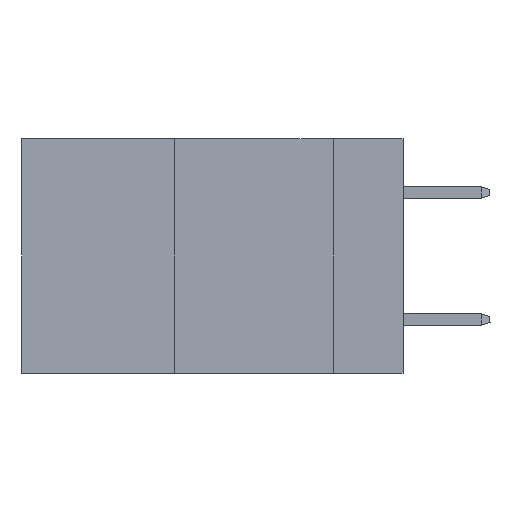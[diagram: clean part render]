
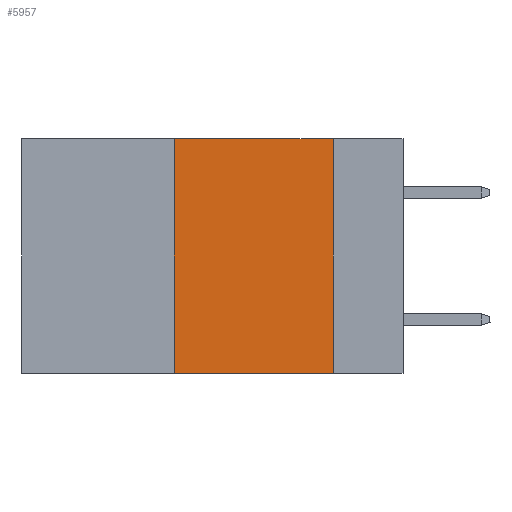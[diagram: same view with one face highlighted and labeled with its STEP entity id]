
A CAD part, left-side view. The second image highlights one B-rep face of the part: STEP entity #5957.
In plain terms, the highlighted planar face has unit normal (-1, 0, 0).
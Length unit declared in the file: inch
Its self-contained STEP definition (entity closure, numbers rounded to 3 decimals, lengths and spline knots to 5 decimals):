
#742 = CARTESIAN_POINT ( 'NONE',  ( 0., 0.6, -0.37 ) ) ;
#1434 = EDGE_CURVE ( 'NONE', #24306, #23493, #7871, .T. ) ;
#1919 = CARTESIAN_POINT ( 'NONE',  ( 0., 0.11, -0.37 ) ) ;
#2840 = DIRECTION ( 'NONE',  ( 0., -1., 0. ) ) ;
#4741 = DIRECTION ( 'NONE',  ( 1., 0., 0. ) ) ;
#4918 = CARTESIAN_POINT ( 'NONE',  ( 0., 0.11, 0. ) ) ;
#5442 = ORIENTED_EDGE ( 'NONE', *, *, #32337, .F. ) ;
#5957 = ADVANCED_FACE ( 'NONE', ( #20159 ), #32544, .F. ) ;
#7871 = LINE ( 'NONE', #13069, #31113 ) ;
#9867 = AXIS2_PLACEMENT_3D ( 'NONE', #14803, #4741, #20486 ) ;
#10451 = DIRECTION ( 'NONE',  ( 0., -1., 0. ) ) ;
#11065 = CARTESIAN_POINT ( 'NONE',  ( 0., 0.11, 0. ) ) ;
#12007 = EDGE_CURVE ( 'NONE', #17244, #28889, #23196, .T. ) ;
#13069 = CARTESIAN_POINT ( 'NONE',  ( 0., 0.6, 0. ) ) ;
#13673 = DIRECTION ( 'NONE',  ( 0., 0., 1. ) ) ;
#14803 = CARTESIAN_POINT ( 'NONE',  ( 0., 0.6, 0. ) ) ;
#17109 = ORIENTED_EDGE ( 'NONE', *, *, #17417, .F. ) ;
#17244 = VERTEX_POINT ( 'NONE', #17950 ) ;
#17417 = EDGE_CURVE ( 'NONE', #23493, #28889, #31646, .T. ) ;
#17438 = VECTOR ( 'NONE', #10451, 39.37008 ) ;
#17950 = CARTESIAN_POINT ( 'NONE',  ( 0., 0.36, -0.37 ) ) ;
#18439 = DIRECTION ( 'NONE',  ( 0., 0., -1. ) ) ;
#20159 = FACE_OUTER_BOUND ( 'NONE', #28668, .T. ) ;
#20486 = DIRECTION ( 'NONE',  ( 0., 0., -1. ) ) ;
#20908 = CARTESIAN_POINT ( 'NONE',  ( 0., 0.36, 0. ) ) ;
#22554 = VECTOR ( 'NONE', #13673, 39.37008 ) ;
#23196 = LINE ( 'NONE', #742, #17438 ) ;
#23493 = VERTEX_POINT ( 'NONE', #4918 ) ;
#23578 = LINE ( 'NONE', #20908, #22554 ) ;
#24306 = VERTEX_POINT ( 'NONE', #29304 ) ;
#28668 = EDGE_LOOP ( 'NONE', ( #17109, #29161, #5442, #31416 ) ) ;
#28889 = VERTEX_POINT ( 'NONE', #1919 ) ;
#29161 = ORIENTED_EDGE ( 'NONE', *, *, #1434, .F. ) ;
#29304 = CARTESIAN_POINT ( 'NONE',  ( 0., 0.36, 0. ) ) ;
#30971 = VECTOR ( 'NONE', #18439, 39.37008 ) ;
#31113 = VECTOR ( 'NONE', #2840, 39.37008 ) ;
#31416 = ORIENTED_EDGE ( 'NONE', *, *, #12007, .T. ) ;
#31646 = LINE ( 'NONE', #11065, #30971 ) ;
#32337 = EDGE_CURVE ( 'NONE', #17244, #24306, #23578, .T. ) ;
#32544 = PLANE ( 'NONE',  #9867 ) ;
